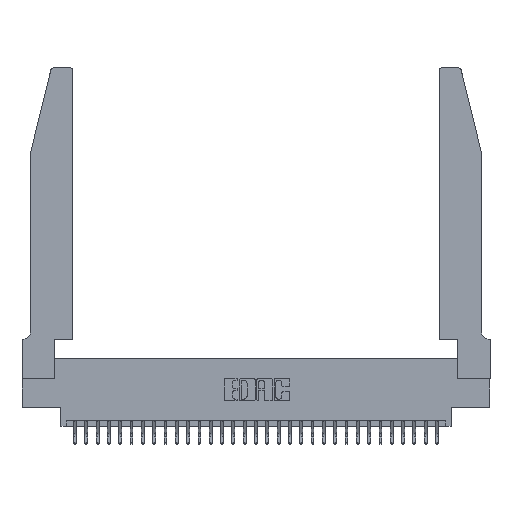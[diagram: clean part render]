
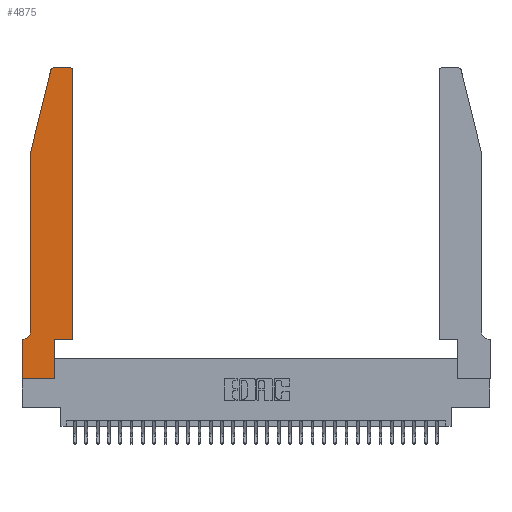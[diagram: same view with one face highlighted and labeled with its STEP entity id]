
A CAD part, top view. The second image highlights one B-rep face of the part: STEP entity #4875.
In plain terms, the highlighted planar face has unit normal (0, 0, 1).
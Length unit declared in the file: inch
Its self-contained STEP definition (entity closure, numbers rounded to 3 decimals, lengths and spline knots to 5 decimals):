
#67 = CARTESIAN_POINT ( 'NONE',  ( 0.2865, 0.35, 0.37 ) ) ;
#274 = DIRECTION ( 'NONE',  ( -1., 0., 0. ) ) ;
#279 = LINE ( 'NONE', #17117, #31827 ) ;
#440 = CARTESIAN_POINT ( 'NONE',  ( 0.0755, 2., 0.37 ) ) ;
#1110 = ORIENTED_EDGE ( 'NONE', *, *, #28363, .T. ) ;
#1525 = VECTOR ( 'NONE', #13115, 39.37008 ) ;
#1666 = CARTESIAN_POINT ( 'NONE',  ( 0.4205, 2.72, 0.37 ) ) ;
#2160 = VERTEX_POINT ( 'NONE', #30915 ) ;
#2670 = VERTEX_POINT ( 'NONE', #28416 ) ;
#2684 = CARTESIAN_POINT ( 'NONE',  ( 0.0755, 0.35, 0.37 ) ) ;
#3051 = ORIENTED_EDGE ( 'NONE', *, *, #23951, .T. ) ;
#3557 = LINE ( 'NONE', #14406, #16964 ) ;
#4183 = DIRECTION ( 'NONE',  ( 1., 0., 0. ) ) ;
#4536 = CARTESIAN_POINT ( 'NONE',  ( 0.2865, 0., 0.37 ) ) ;
#4875 = ADVANCED_FACE ( 'NONE', ( #15498 ), #14902, .T. ) ;
#4876 = DIRECTION ( 'NONE',  ( 1., 0., 0. ) ) ;
#5130 = LINE ( 'NONE', #5809, #6713 ) ;
#5809 = CARTESIAN_POINT ( 'NONE',  ( 0.4505, 0.35, 0.37 ) ) ;
#6294 = CIRCLE ( 'NONE', #16199, 0.03 ) ;
#6713 = VECTOR ( 'NONE', #23244, 39.37008 ) ;
#6740 = DIRECTION ( 'NONE',  ( 0., 1., 0. ) ) ;
#7004 = DIRECTION ( 'NONE',  ( 0., -1., 0. ) ) ;
#7056 = DIRECTION ( 'NONE',  ( -0.239, -0.971, 0. ) ) ;
#8275 = CARTESIAN_POINT ( 'NONE',  ( 0.284, 2.72, 0.37 ) ) ;
#9290 = EDGE_CURVE ( 'NONE', #2670, #32062, #19055, .T. ) ;
#10402 = ORIENTED_EDGE ( 'NONE', *, *, #9290, .T. ) ;
#10781 = DIRECTION ( 'NONE',  ( 1., 0., 0. ) ) ;
#10847 = VERTEX_POINT ( 'NONE', #21027 ) ;
#11429 = ORIENTED_EDGE ( 'NONE', *, *, #26142, .T. ) ;
#11488 = CARTESIAN_POINT ( 'NONE',  ( 0.0055, 0.35, 0.37 ) ) ;
#11576 = ORIENTED_EDGE ( 'NONE', *, *, #18153, .T. ) ;
#11660 = CARTESIAN_POINT ( 'NONE',  ( 0.2865, 0.35, 0.37 ) ) ;
#11684 = VERTEX_POINT ( 'NONE', #12275 ) ;
#12275 = CARTESIAN_POINT ( 'NONE',  ( 0.4505, 0.35, 0.37 ) ) ;
#12340 = CARTESIAN_POINT ( 'NONE',  ( 0., 0.35, 0.37 ) ) ;
#12729 = VERTEX_POINT ( 'NONE', #29822 ) ;
#13115 = DIRECTION ( 'NONE',  ( 1., 0., 0. ) ) ;
#13193 = CIRCLE ( 'NONE', #29123, 0.03 ) ;
#14035 = DIRECTION ( 'NONE',  ( 0., 0., -1. ) ) ;
#14054 = ORIENTED_EDGE ( 'NONE', *, *, #23453, .T. ) ;
#14340 = ORIENTED_EDGE ( 'NONE', *, *, #20034, .T. ) ;
#14406 = CARTESIAN_POINT ( 'NONE',  ( 0.4505, 0.35, 0.37 ) ) ;
#14902 = PLANE ( 'NONE',  #22093 ) ;
#15498 = FACE_OUTER_BOUND ( 'NONE', #17573, .T. ) ;
#15703 = LINE ( 'NONE', #25465, #1525 ) ;
#15713 = ORIENTED_EDGE ( 'NONE', *, *, #23861, .T. ) ;
#16199 = AXIS2_PLACEMENT_3D ( 'NONE', #8275, #25682, #10781 ) ;
#16435 = ORIENTED_EDGE ( 'NONE', *, *, #20920, .T. ) ;
#16622 = VERTEX_POINT ( 'NONE', #22430 ) ;
#16665 = LINE ( 'NONE', #440, #28976 ) ;
#16933 = LINE ( 'NONE', #2684, #22706 ) ;
#16964 = VECTOR ( 'NONE', #26733, 39.37008 ) ;
#17117 = CARTESIAN_POINT ( 'NONE',  ( 0., 0., 0.37 ) ) ;
#17573 = EDGE_LOOP ( 'NONE', ( #16435, #22928, #10402, #31334, #20856, #3051, #1110, #11576, #11429, #14054, #15713, #14340 ) ) ;
#18153 = EDGE_CURVE ( 'NONE', #16622, #19651, #15703, .T. ) ;
#18923 = VERTEX_POINT ( 'NONE', #11488 ) ;
#19055 = LINE ( 'NONE', #21997, #25593 ) ;
#19216 = DIRECTION ( 'NONE',  ( 0., 0., 1. ) ) ;
#19651 = VERTEX_POINT ( 'NONE', #4536 ) ;
#19659 = VECTOR ( 'NONE', #6740, 39.37008 ) ;
#19898 = DIRECTION ( 'NONE',  ( 0., 0., 1. ) ) ;
#20034 = EDGE_CURVE ( 'NONE', #30820, #2160, #13193, .T. ) ;
#20231 = DIRECTION ( 'NONE',  ( -1., 0., 0. ) ) ;
#20856 = ORIENTED_EDGE ( 'NONE', *, *, #30276, .T. ) ;
#20920 = EDGE_CURVE ( 'NONE', #2160, #12729, #27525, .T. ) ;
#20956 = VECTOR ( 'NONE', #20231, 39.37008 ) ;
#21027 = CARTESIAN_POINT ( 'NONE',  ( 0.0755, 0.42, 0.37 ) ) ;
#21997 = CARTESIAN_POINT ( 'NONE',  ( 0.0755, 2., 0.37 ) ) ;
#22093 = AXIS2_PLACEMENT_3D ( 'NONE', #12340, #19898, #4876 ) ;
#22430 = CARTESIAN_POINT ( 'NONE',  ( 0., 0., 0.37 ) ) ;
#22593 = VERTEX_POINT ( 'NONE', #67 ) ;
#22706 = VECTOR ( 'NONE', #274, 39.37008 ) ;
#22928 = ORIENTED_EDGE ( 'NONE', *, *, #24068, .T. ) ;
#22944 = DIRECTION ( 'NONE',  ( 0., -1., 0. ) ) ;
#23244 = DIRECTION ( 'NONE',  ( 0., 1., 0. ) ) ;
#23453 = EDGE_CURVE ( 'NONE', #22593, #11684, #3557, .T. ) ;
#23861 = EDGE_CURVE ( 'NONE', #11684, #30820, #5130, .T. ) ;
#23951 = EDGE_CURVE ( 'NONE', #18923, #30116, #16933, .T. ) ;
#24068 = EDGE_CURVE ( 'NONE', #12729, #2670, #6294, .T. ) ;
#25465 = CARTESIAN_POINT ( 'NONE',  ( 0., 0., 0.37 ) ) ;
#25593 = VECTOR ( 'NONE', #7056, 39.37008 ) ;
#25682 = DIRECTION ( 'NONE',  ( 0., 0., 1. ) ) ;
#26142 = EDGE_CURVE ( 'NONE', #19651, #22593, #31190, .T. ) ;
#26282 = CARTESIAN_POINT ( 'NONE',  ( 0.0755, 2., 0.37 ) ) ;
#26733 = DIRECTION ( 'NONE',  ( 1., 0., 0. ) ) ;
#27525 = LINE ( 'NONE', #30007, #20956 ) ;
#28211 = CARTESIAN_POINT ( 'NONE',  ( 0., 0.35, 0.37 ) ) ;
#28257 = CIRCLE ( 'NONE', #31202, 0.07 ) ;
#28363 = EDGE_CURVE ( 'NONE', #30116, #16622, #279, .T. ) ;
#28416 = CARTESIAN_POINT ( 'NONE',  ( 0.25487, 2.72718, 0.37 ) ) ;
#28831 = CARTESIAN_POINT ( 'NONE',  ( 0.0055, 0.42, 0.37 ) ) ;
#28976 = VECTOR ( 'NONE', #22944, 39.37008 ) ;
#29123 = AXIS2_PLACEMENT_3D ( 'NONE', #1666, #19216, #4183 ) ;
#29822 = CARTESIAN_POINT ( 'NONE',  ( 0.284, 2.75, 0.37 ) ) ;
#30007 = CARTESIAN_POINT ( 'NONE',  ( 0.2605, 2.75, 0.37 ) ) ;
#30021 = EDGE_CURVE ( 'NONE', #32062, #10847, #16665, .T. ) ;
#30116 = VERTEX_POINT ( 'NONE', #28211 ) ;
#30276 = EDGE_CURVE ( 'NONE', #10847, #18923, #28257, .T. ) ;
#30627 = CARTESIAN_POINT ( 'NONE',  ( 0.4505, 2.72, 0.37 ) ) ;
#30820 = VERTEX_POINT ( 'NONE', #30627 ) ;
#30915 = CARTESIAN_POINT ( 'NONE',  ( 0.4205, 2.75, 0.37 ) ) ;
#31190 = LINE ( 'NONE', #11660, #19659 ) ;
#31202 = AXIS2_PLACEMENT_3D ( 'NONE', #28831, #14035, #31326 ) ;
#31326 = DIRECTION ( 'NONE',  ( -1., 0., 0. ) ) ;
#31334 = ORIENTED_EDGE ( 'NONE', *, *, #30021, .T. ) ;
#31827 = VECTOR ( 'NONE', #7004, 39.37008 ) ;
#32062 = VERTEX_POINT ( 'NONE', #26282 ) ;
